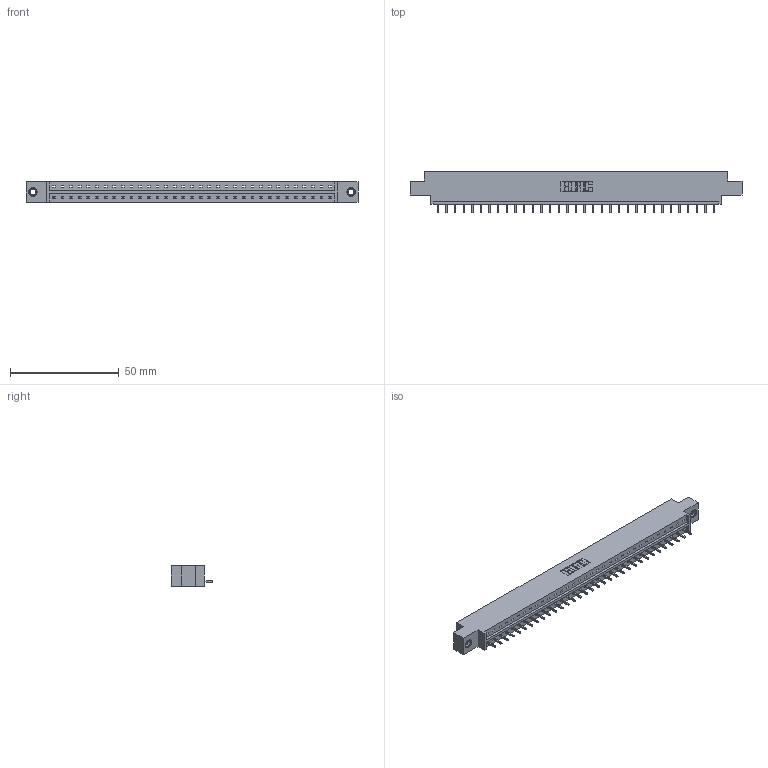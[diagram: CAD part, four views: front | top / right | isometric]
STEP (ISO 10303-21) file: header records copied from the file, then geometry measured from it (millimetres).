
FILE_DESCRIPTION (( 'STEP AP203' ), '1' );
FILE_NAME ('833-033-521-607.STEP', '2020-06-02T19:57:15', ( '' ), ( '' ), 'SwSTEP 2.0', 'SolidWorks 2020', '' );
FILE_SCHEMA (( 'CONFIG_CONTROL_DESIGN' ));
Length unit declared in the file: inch
Products named in the file (4): 833 Part_Offset - .156 Dia - TI; 833-033-521-607; 345-250-001_345-250-005-103; 345-292-001_345-293-121
Assembly tree (36 placements, depth 2):
  833-033-521-607
    833 Part_Offset - .156 Dia - TI
    345-292-001_345-293-121  x33
    345-250-001_345-250-005-103  x2
Bounding box: 152.3 x 19.06 x 9.4 mm (x, y, z)
Volume: 14912.9 mm3; surface area: 15922.8 mm2
Topology: 36 solids, 36 shells, 2092 faces, 6267 edges, 4126 vertices
Faces by surface type: plane 1492, cylinder 584, cone 12, torus 4
Entity records: 22674 total; most frequent: CARTESIAN_POINT 3896, ORIENTED_EDGE 3858, DIRECTION 3337, EDGE_CURVE 1929, LINE 1781, VECTOR 1781, VERTEX_POINT 1280, AXIS2_PLACEMENT_3D 778
